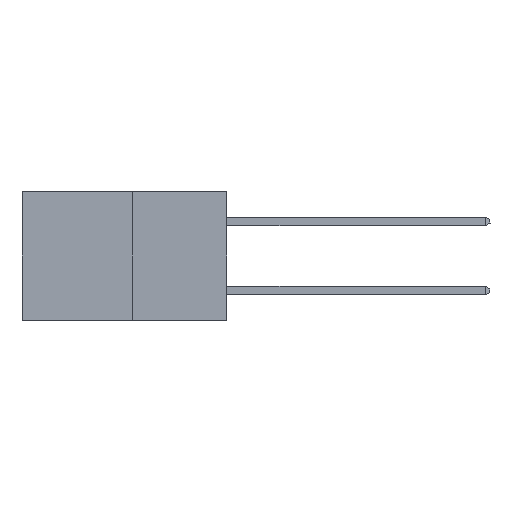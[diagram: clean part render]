
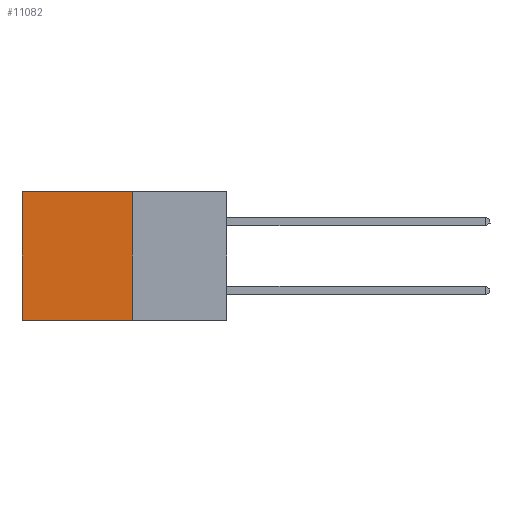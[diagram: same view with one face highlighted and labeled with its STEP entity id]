
A CAD part, left-side view. The second image highlights one B-rep face of the part: STEP entity #11082.
In plain terms, the highlighted planar face has unit normal (-1, 0, 0).
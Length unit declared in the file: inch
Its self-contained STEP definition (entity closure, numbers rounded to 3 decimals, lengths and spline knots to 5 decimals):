
#277 = DIRECTION ( 'NONE',  ( 0., 1., 0. ) ) ;
#1626 = EDGE_LOOP ( 'NONE', ( #3362, #5008, #2047, #3375 ) ) ;
#1645 = VECTOR ( 'NONE', #277, 39.37008 ) ;
#2047 = ORIENTED_EDGE ( 'NONE', *, *, #7862, .F. ) ;
#2093 = EDGE_CURVE ( 'NONE', #3849, #11097, #11417, .T. ) ;
#2277 = CARTESIAN_POINT ( 'NONE',  ( 0.277, 0.27, 0. ) ) ;
#2575 = VERTEX_POINT ( 'NONE', #5196 ) ;
#2609 = DIRECTION ( 'NONE',  ( 0., 0., -1. ) ) ;
#2650 = CARTESIAN_POINT ( 'NONE',  ( 0.277, 0.59, -0.37 ) ) ;
#2826 = CARTESIAN_POINT ( 'NONE',  ( 0.277, 0.59, 0. ) ) ;
#3208 = CARTESIAN_POINT ( 'NONE',  ( 0.277, 0.59, -0.37 ) ) ;
#3362 = ORIENTED_EDGE ( 'NONE', *, *, #2093, .T. ) ;
#3375 = ORIENTED_EDGE ( 'NONE', *, *, #10158, .T. ) ;
#3849 = VERTEX_POINT ( 'NONE', #2826 ) ;
#4322 = VECTOR ( 'NONE', #6574, 39.37008 ) ;
#4410 = DIRECTION ( 'NONE',  ( 0., 1., 0. ) ) ;
#4605 = VECTOR ( 'NONE', #8187, 39.37008 ) ;
#5008 = ORIENTED_EDGE ( 'NONE', *, *, #9137, .F. ) ;
#5196 = CARTESIAN_POINT ( 'NONE',  ( 0.277, 0.27, -0.37 ) ) ;
#5612 = CARTESIAN_POINT ( 'NONE',  ( 0.277, 0.27, -0.37 ) ) ;
#5616 = VECTOR ( 'NONE', #4410, 39.37008 ) ;
#6574 = DIRECTION ( 'NONE',  ( 0., 0., -1. ) ) ;
#6601 = LINE ( 'NONE', #10915, #1645 ) ;
#6983 = VERTEX_POINT ( 'NONE', #2277 ) ;
#7443 = AXIS2_PLACEMENT_3D ( 'NONE', #9684, #8018, #2609 ) ;
#7672 = LINE ( 'NONE', #9653, #5616 ) ;
#7862 = EDGE_CURVE ( 'NONE', #6983, #2575, #8995, .T. ) ;
#8018 = DIRECTION ( 'NONE',  ( 1., 0., 0. ) ) ;
#8187 = DIRECTION ( 'NONE',  ( 0., 0., -1. ) ) ;
#8995 = LINE ( 'NONE', #5612, #4605 ) ;
#9137 = EDGE_CURVE ( 'NONE', #2575, #11097, #7672, .T. ) ;
#9653 = CARTESIAN_POINT ( 'NONE',  ( 0.277, 0.27, -0.37 ) ) ;
#9684 = CARTESIAN_POINT ( 'NONE',  ( 0.277, 0.27, -0.37 ) ) ;
#9976 = FACE_OUTER_BOUND ( 'NONE', #1626, .T. ) ;
#10158 = EDGE_CURVE ( 'NONE', #6983, #3849, #6601, .T. ) ;
#10915 = CARTESIAN_POINT ( 'NONE',  ( 0.277, 0.27, 0. ) ) ;
#11082 = ADVANCED_FACE ( 'NONE', ( #9976 ), #11286, .F. ) ;
#11097 = VERTEX_POINT ( 'NONE', #2650 ) ;
#11286 = PLANE ( 'NONE',  #7443 ) ;
#11417 = LINE ( 'NONE', #3208, #4322 ) ;
